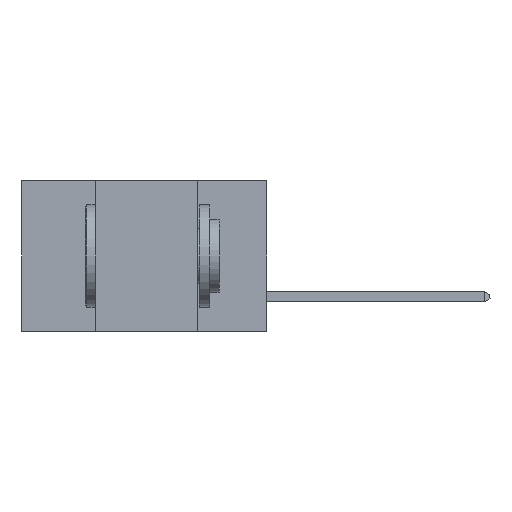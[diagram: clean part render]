
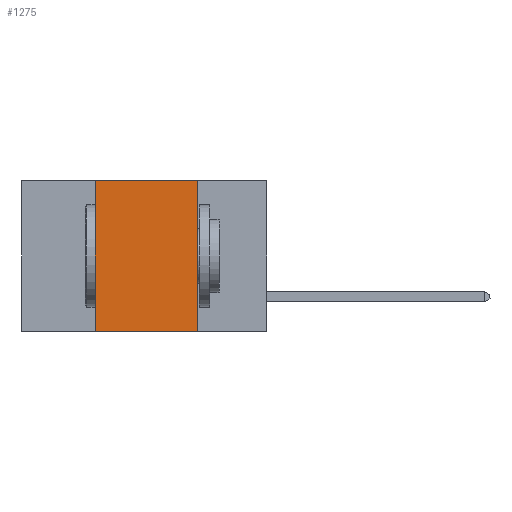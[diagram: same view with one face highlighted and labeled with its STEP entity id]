
A CAD part, left-side view. The second image highlights one B-rep face of the part: STEP entity #1275.
In plain terms, the highlighted planar face has unit normal (-1, 0, 0).
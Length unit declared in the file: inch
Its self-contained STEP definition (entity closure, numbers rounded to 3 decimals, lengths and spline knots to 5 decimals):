
#266 = ORIENTED_EDGE ( 'NONE', *, *, #734, .T. ) ;
#734 = EDGE_CURVE ( 'NONE', #10091, #13246, #16335, .T. ) ;
#740 = DIRECTION ( 'NONE',  ( 0., -1., 0. ) ) ;
#789 = VECTOR ( 'NONE', #3220, 39.37008 ) ;
#832 = EDGE_CURVE ( 'NONE', #10091, #16921, #8693, .T. ) ;
#899 = AXIS2_PLACEMENT_3D ( 'NONE', #9126, #2994, #15841 ) ;
#1014 = EDGE_CURVE ( 'NONE', #5832, #13246, #12258, .T. ) ;
#1275 = ADVANCED_FACE ( 'NONE', ( #6524 ), #8383, .F. ) ;
#1504 = VECTOR ( 'NONE', #7678, 39.37008 ) ;
#2994 = DIRECTION ( 'NONE',  ( 1., 0., 0. ) ) ;
#3220 = DIRECTION ( 'NONE',  ( 0., 0., 1. ) ) ;
#3289 = EDGE_CURVE ( 'NONE', #16921, #5832, #7952, .T. ) ;
#3918 = ORIENTED_EDGE ( 'NONE', *, *, #3289, .F. ) ;
#5146 = CARTESIAN_POINT ( 'NONE',  ( 0., 0.17, 0. ) ) ;
#5832 = VERTEX_POINT ( 'NONE', #5146 ) ;
#5921 = CARTESIAN_POINT ( 'NONE',  ( 0., 0.42, 0. ) ) ;
#6524 = FACE_OUTER_BOUND ( 'NONE', #7573, .T. ) ;
#6906 = ORIENTED_EDGE ( 'NONE', *, *, #1014, .F. ) ;
#7573 = EDGE_LOOP ( 'NONE', ( #6906, #3918, #12896, #266 ) ) ;
#7678 = DIRECTION ( 'NONE',  ( 0., 0., -1. ) ) ;
#7751 = CARTESIAN_POINT ( 'NONE',  ( 0., 0.17, 0. ) ) ;
#7952 = LINE ( 'NONE', #12754, #14204 ) ;
#8383 = PLANE ( 'NONE',  #899 ) ;
#8693 = LINE ( 'NONE', #15449, #789 ) ;
#9072 = CARTESIAN_POINT ( 'NONE',  ( 0., 0.6, -0.37 ) ) ;
#9126 = CARTESIAN_POINT ( 'NONE',  ( 0., 0.6, 0. ) ) ;
#10091 = VERTEX_POINT ( 'NONE', #13179 ) ;
#12258 = LINE ( 'NONE', #7751, #1504 ) ;
#12459 = VECTOR ( 'NONE', #740, 39.37008 ) ;
#12723 = DIRECTION ( 'NONE',  ( 0., -1., 0. ) ) ;
#12754 = CARTESIAN_POINT ( 'NONE',  ( 0., 0.6, 0. ) ) ;
#12896 = ORIENTED_EDGE ( 'NONE', *, *, #832, .F. ) ;
#13088 = CARTESIAN_POINT ( 'NONE',  ( 0., 0.17, -0.37 ) ) ;
#13179 = CARTESIAN_POINT ( 'NONE',  ( 0., 0.42, -0.37 ) ) ;
#13246 = VERTEX_POINT ( 'NONE', #13088 ) ;
#14204 = VECTOR ( 'NONE', #12723, 39.37008 ) ;
#15449 = CARTESIAN_POINT ( 'NONE',  ( 0., 0.42, 0. ) ) ;
#15841 = DIRECTION ( 'NONE',  ( 0., 0., -1. ) ) ;
#16335 = LINE ( 'NONE', #9072, #12459 ) ;
#16921 = VERTEX_POINT ( 'NONE', #5921 ) ;
